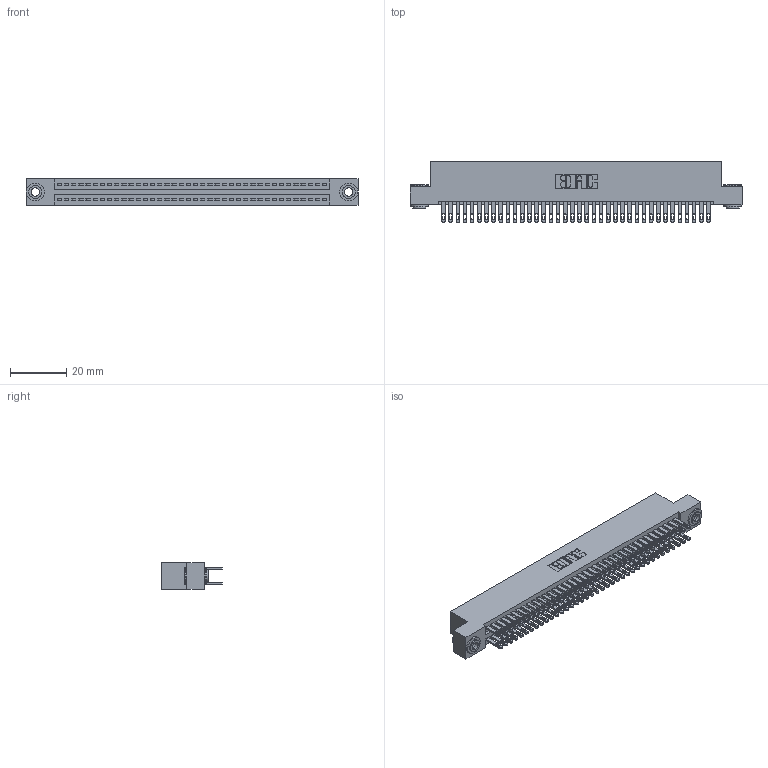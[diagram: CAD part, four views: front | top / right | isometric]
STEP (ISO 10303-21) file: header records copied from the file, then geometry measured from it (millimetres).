
FILE_DESCRIPTION (( 'STEP AP203' ), '1' );
FILE_NAME ('345-076-500-203.STEP', '2018-10-02T14:38:54', ( '' ), ( '' ), 'SwSTEP 2.0', 'SolidWorks 2016', '' );
FILE_SCHEMA (( 'CONFIG_CONTROL_DESIGN' ));
Length unit declared in the file: inch
Products named in the file (4): 345-076-500-203; 345-250-002_345-250-002-102; 345 Part_Flush Mounting Lugs - 0.156 Dia-TH; 345-292-001_345-293-100
Assembly tree (79 placements, depth 2):
  345-076-500-203
    345 Part_Flush Mounting Lugs - 0.156 Dia-TH
    345-292-001_345-293-100  x76
    345-250-002_345-250-002-102  x2
Bounding box: 117.73 x 21.51 x 9.4 mm (x, y, z)
Volume: 11650.8 mm3; surface area: 18124.5 mm2
Topology: 79 solids, 79 shells, 3660 faces, 11133 edges, 7418 vertices
Faces by surface type: plane 2142, cylinder 1510, cone 8
Entity records: 30934 total; most frequent: CARTESIAN_POINT 5163, ORIENTED_EDGE 5090, DIRECTION 4591, EDGE_CURVE 2545, LINE 2233, VECTOR 2233, VERTEX_POINT 1694, AXIS2_PLACEMENT_3D 1179
